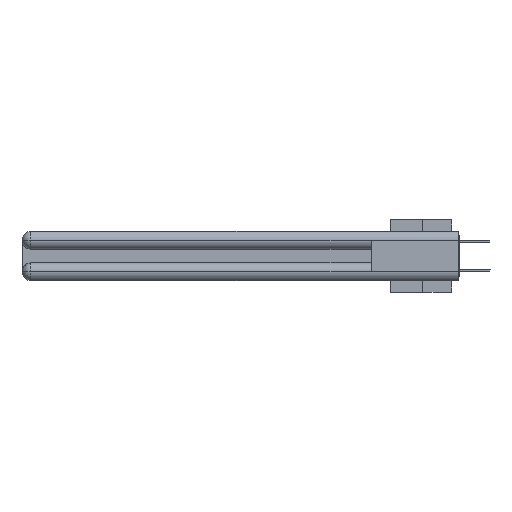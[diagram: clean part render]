
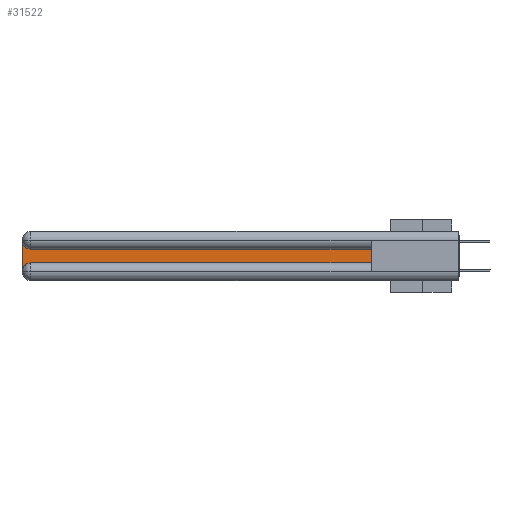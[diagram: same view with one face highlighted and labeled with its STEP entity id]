
A CAD part, left-side view. The second image highlights one B-rep face of the part: STEP entity #31522.
In plain terms, the highlighted planar face has unit normal (-1, 0, 0).
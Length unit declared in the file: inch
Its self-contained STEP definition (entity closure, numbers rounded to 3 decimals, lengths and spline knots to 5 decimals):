
#965 = VERTEX_POINT ( 'NONE', #2950 ) ;
#2260 = VERTEX_POINT ( 'NONE', #2420 ) ;
#2319 = CARTESIAN_POINT ( 'NONE',  ( 0.075, 0.6, -0.2175 ) ) ;
#2420 = CARTESIAN_POINT ( 'NONE',  ( 0.075, 3., -0.2775 ) ) ;
#2687 = DIRECTION ( 'NONE',  ( 0., 0., 1. ) ) ;
#2950 = CARTESIAN_POINT ( 'NONE',  ( 0.075, 2.94, -0.2175 ) ) ;
#3216 = EDGE_LOOP ( 'NONE', ( #5823, #22964, #14955, #12718, #20112, #23615 ) ) ;
#3925 = VERTEX_POINT ( 'NONE', #22415 ) ;
#3928 = DIRECTION ( 'NONE',  ( 1., 0., 0. ) ) ;
#4474 = FACE_OUTER_BOUND ( 'NONE', #3216, .T. ) ;
#4569 = EDGE_CURVE ( 'NONE', #16551, #26110, #7673, .T. ) ;
#5005 = DIRECTION ( 'NONE',  ( 1., 0., 0. ) ) ;
#5207 = CARTESIAN_POINT ( 'NONE',  ( 0.075, 2.94, -0.2775 ) ) ;
#5431 = AXIS2_PLACEMENT_3D ( 'NONE', #11309, #14047, #9169 ) ;
#5823 = ORIENTED_EDGE ( 'NONE', *, *, #20497, .T. ) ;
#6049 = DIRECTION ( 'NONE',  ( 0., 0., -1. ) ) ;
#6123 = DIRECTION ( 'NONE',  ( 0., -1., 0. ) ) ;
#6742 = VECTOR ( 'NONE', #6049, 39.37008 ) ;
#7316 = VECTOR ( 'NONE', #2687, 39.37008 ) ;
#7673 = LINE ( 'NONE', #14815, #7316 ) ;
#8396 = DIRECTION ( 'NONE',  ( 0., 0., -1. ) ) ;
#9169 = DIRECTION ( 'NONE',  ( 0., 0., -1. ) ) ;
#9368 = AXIS2_PLACEMENT_3D ( 'NONE', #5207, #5005, #22220 ) ;
#10927 = CARTESIAN_POINT ( 'NONE',  ( 0.075, 3., -0.2175 ) ) ;
#10957 = CARTESIAN_POINT ( 'NONE',  ( 0.075, 3., -0.1225 ) ) ;
#11309 = CARTESIAN_POINT ( 'NONE',  ( 0.075, 2.94, -0.0625 ) ) ;
#12705 = EDGE_CURVE ( 'NONE', #3925, #27166, #13790, .T. ) ;
#12718 = ORIENTED_EDGE ( 'NONE', *, *, #24211, .T. ) ;
#13593 = CARTESIAN_POINT ( 'NONE',  ( 0.075, 3., -0.0625 ) ) ;
#13790 = CIRCLE ( 'NONE', #5431, 0.06 ) ;
#14047 = DIRECTION ( 'NONE',  ( 1., 0., 0. ) ) ;
#14164 = DIRECTION ( 'NONE',  ( 0., 1., 0. ) ) ;
#14815 = CARTESIAN_POINT ( 'NONE',  ( 0.075, 0.6, -0.2175 ) ) ;
#14955 = ORIENTED_EDGE ( 'NONE', *, *, #30089, .T. ) ;
#15545 = VECTOR ( 'NONE', #14164, 39.37008 ) ;
#15782 = AXIS2_PLACEMENT_3D ( 'NONE', #10957, #3928, #8396 ) ;
#15944 = PLANE ( 'NONE',  #15782 ) ;
#16177 = VECTOR ( 'NONE', #6123, 39.37008 ) ;
#16505 = CARTESIAN_POINT ( 'NONE',  ( 0.075, 0.6, -0.1225 ) ) ;
#16551 = VERTEX_POINT ( 'NONE', #2319 ) ;
#16947 = CARTESIAN_POINT ( 'NONE',  ( 0.075, 0.6, -0.1225 ) ) ;
#16964 = EDGE_CURVE ( 'NONE', #965, #16551, #21898, .T. ) ;
#19734 = LINE ( 'NONE', #16505, #15545 ) ;
#20112 = ORIENTED_EDGE ( 'NONE', *, *, #16964, .T. ) ;
#20497 = EDGE_CURVE ( 'NONE', #26110, #3925, #19734, .T. ) ;
#21898 = LINE ( 'NONE', #27854, #16177 ) ;
#22220 = DIRECTION ( 'NONE',  ( 0., 0., -1. ) ) ;
#22415 = CARTESIAN_POINT ( 'NONE',  ( 0.075, 2.94, -0.1225 ) ) ;
#22964 = ORIENTED_EDGE ( 'NONE', *, *, #12705, .T. ) ;
#23615 = ORIENTED_EDGE ( 'NONE', *, *, #4569, .T. ) ;
#24211 = EDGE_CURVE ( 'NONE', #2260, #965, #29423, .T. ) ;
#26110 = VERTEX_POINT ( 'NONE', #16947 ) ;
#27166 = VERTEX_POINT ( 'NONE', #13593 ) ;
#27854 = CARTESIAN_POINT ( 'NONE',  ( 0.075, 0.6, -0.2175 ) ) ;
#28468 = LINE ( 'NONE', #10927, #6742 ) ;
#29423 = CIRCLE ( 'NONE', #9368, 0.06 ) ;
#30089 = EDGE_CURVE ( 'NONE', #27166, #2260, #28468, .T. ) ;
#31522 = ADVANCED_FACE ( 'NONE', ( #4474 ), #15944, .F. ) ;
